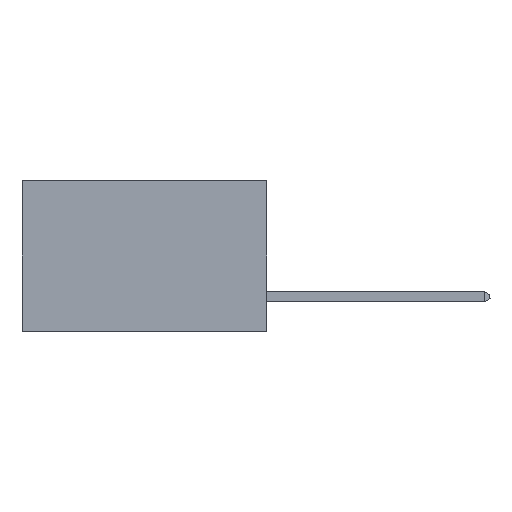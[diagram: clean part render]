
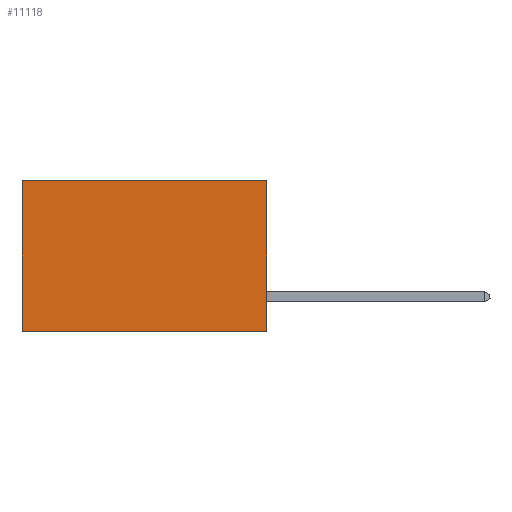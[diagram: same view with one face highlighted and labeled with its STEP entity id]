
A CAD part, left-side view. The second image highlights one B-rep face of the part: STEP entity #11118.
In plain terms, the highlighted planar face has unit normal (-1, 0, 0).
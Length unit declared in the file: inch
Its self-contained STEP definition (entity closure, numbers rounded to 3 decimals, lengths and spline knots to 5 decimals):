
#57 = CARTESIAN_POINT ( 'NONE',  ( 0.2875, 0.6, 0. ) ) ;
#226 = VERTEX_POINT ( 'NONE', #2125 ) ;
#246 = ORIENTED_EDGE ( 'NONE', *, *, #6338, .F. ) ;
#832 = LINE ( 'NONE', #57, #1582 ) ;
#841 = LINE ( 'NONE', #4126, #6233 ) ;
#1019 = DIRECTION ( 'NONE',  ( 0., 0., -1. ) ) ;
#1203 = VERTEX_POINT ( 'NONE', #10294 ) ;
#1265 = EDGE_CURVE ( 'NONE', #2951, #10502, #11606, .T. ) ;
#1383 = CARTESIAN_POINT ( 'NONE',  ( 0.2875, 0., 0. ) ) ;
#1506 = CARTESIAN_POINT ( 'NONE',  ( 0.2875, 0., 0. ) ) ;
#1582 = VECTOR ( 'NONE', #1019, 39.37008 ) ;
#2044 = CARTESIAN_POINT ( 'NONE',  ( 0.2875, 0., 0. ) ) ;
#2125 = CARTESIAN_POINT ( 'NONE',  ( 0.2875, 0.6, -0.37 ) ) ;
#2951 = VERTEX_POINT ( 'NONE', #3045 ) ;
#3045 = CARTESIAN_POINT ( 'NONE',  ( 0.2875, 0., 0. ) ) ;
#3344 = ORIENTED_EDGE ( 'NONE', *, *, #7308, .T. ) ;
#4126 = CARTESIAN_POINT ( 'NONE',  ( 0.2875, 0., -0.37 ) ) ;
#4335 = DIRECTION ( 'NONE',  ( 1., 0., 0. ) ) ;
#5041 = LINE ( 'NONE', #1383, #8170 ) ;
#5142 = DIRECTION ( 'NONE',  ( 0., 1., 0. ) ) ;
#6227 = PLANE ( 'NONE',  #7325 ) ;
#6233 = VECTOR ( 'NONE', #5142, 39.37008 ) ;
#6338 = EDGE_CURVE ( 'NONE', #10502, #226, #841, .T. ) ;
#7015 = FACE_OUTER_BOUND ( 'NONE', #9477, .T. ) ;
#7308 = EDGE_CURVE ( 'NONE', #2951, #1203, #5041, .T. ) ;
#7325 = AXIS2_PLACEMENT_3D ( 'NONE', #1506, #4335, #8948 ) ;
#8170 = VECTOR ( 'NONE', #11751, 39.37008 ) ;
#8948 = DIRECTION ( 'NONE',  ( 0., 0., -1. ) ) ;
#9096 = VECTOR ( 'NONE', #10501, 39.37008 ) ;
#9331 = ORIENTED_EDGE ( 'NONE', *, *, #1265, .F. ) ;
#9477 = EDGE_LOOP ( 'NONE', ( #10161, #246, #9331, #3344 ) ) ;
#10161 = ORIENTED_EDGE ( 'NONE', *, *, #11508, .T. ) ;
#10294 = CARTESIAN_POINT ( 'NONE',  ( 0.2875, 0.6, 0. ) ) ;
#10501 = DIRECTION ( 'NONE',  ( 0., 0., -1. ) ) ;
#10502 = VERTEX_POINT ( 'NONE', #10651 ) ;
#10651 = CARTESIAN_POINT ( 'NONE',  ( 0.2875, 0., -0.37 ) ) ;
#11118 = ADVANCED_FACE ( 'NONE', ( #7015 ), #6227, .F. ) ;
#11508 = EDGE_CURVE ( 'NONE', #1203, #226, #832, .T. ) ;
#11606 = LINE ( 'NONE', #2044, #9096 ) ;
#11751 = DIRECTION ( 'NONE',  ( 0., 1., 0. ) ) ;
